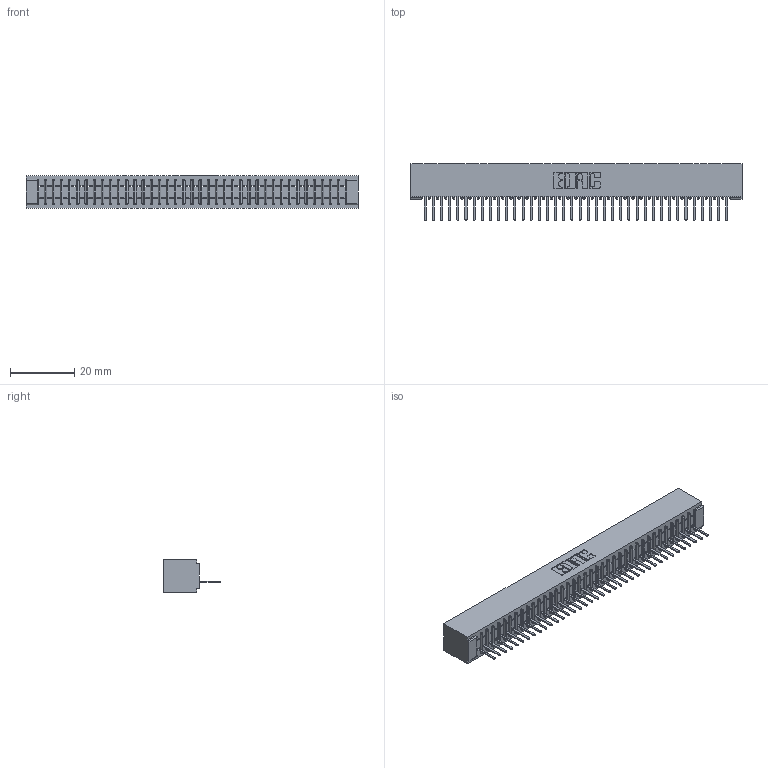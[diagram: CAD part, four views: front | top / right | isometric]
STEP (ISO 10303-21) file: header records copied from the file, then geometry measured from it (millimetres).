
FILE_DESCRIPTION (( 'STEP AP203' ), '1' );
FILE_NAME ('391-038-521-101.STEP', '2018-08-09T00:02:04', ( '' ), ( '' ), 'SwSTEP 2.0', 'SolidWorks 2016', '' );
FILE_SCHEMA (( 'CONFIG_CONTROL_DESIGN' ));
Length unit declared in the file: inch
Products named in the file (3): 341 Part_No Mounting Lugs; 341-292-001_341-292-121; 391-038-521-101
Assembly tree (39 placements, depth 2):
  391-038-521-101
    341 Part_No Mounting Lugs
    341-292-001_341-292-121  x38
Bounding box: 103.5 x 17.7 x 10.16 mm (x, y, z)
Volume: 7632.5 mm3; surface area: 12359.8 mm2
Topology: 39 solids, 39 shells, 3224 faces, 9298 edges, 5966 vertices
Faces by surface type: plane 2002, cylinder 1070, sphere 78, torus 74
Entity records: 45027 total; most frequent: CARTESIAN_POINT 7648, ORIENTED_EDGE 7636, DIRECTION 7384, EDGE_CURVE 3818, LINE 3084, VECTOR 3084, VERTEX_POINT 2414, AXIS2_PLACEMENT_3D 2150
